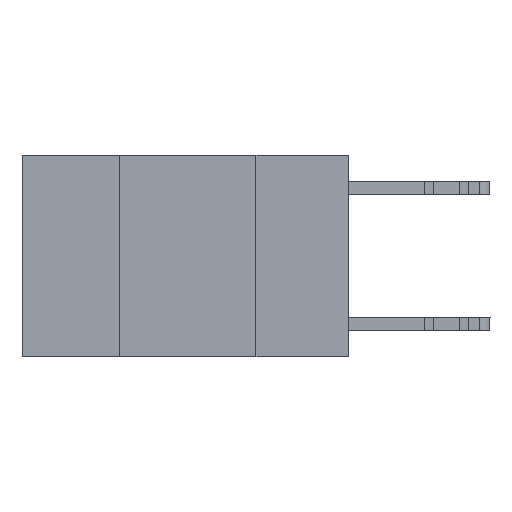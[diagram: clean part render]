
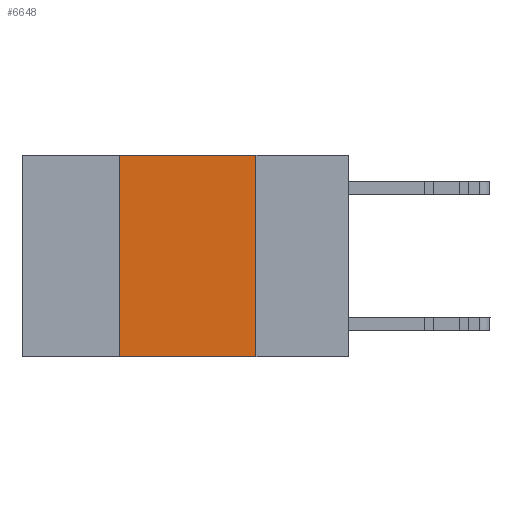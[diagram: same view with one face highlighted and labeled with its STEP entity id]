
A CAD part, left-side view. The second image highlights one B-rep face of the part: STEP entity #6648.
In plain terms, the highlighted planar face has unit normal (-1, 0, 0).
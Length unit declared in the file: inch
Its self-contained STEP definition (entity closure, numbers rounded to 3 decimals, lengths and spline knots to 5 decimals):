
#699 = LINE ( 'NONE', #27373, #13231 ) ;
#2178 = FACE_OUTER_BOUND ( 'NONE', #12333, .T. ) ;
#2464 = VERTEX_POINT ( 'NONE', #16812 ) ;
#3561 = DIRECTION ( 'NONE',  ( 0., 0., 1. ) ) ;
#5407 = VECTOR ( 'NONE', #8042, 39.37008 ) ;
#5435 = LINE ( 'NONE', #5542, #5407 ) ;
#5542 = CARTESIAN_POINT ( 'NONE',  ( 0., 0.17, 0. ) ) ;
#6648 = ADVANCED_FACE ( 'NONE', ( #2178 ), #23026, .F. ) ;
#8042 = DIRECTION ( 'NONE',  ( 0., 0., -1. ) ) ;
#11123 = VERTEX_POINT ( 'NONE', #26654 ) ;
#11436 = EDGE_CURVE ( 'NONE', #31077, #23239, #5435, .T. ) ;
#12333 = EDGE_LOOP ( 'NONE', ( #30022, #15157, #30770, #29256 ) ) ;
#13231 = VECTOR ( 'NONE', #15193, 39.37008 ) ;
#15157 = ORIENTED_EDGE ( 'NONE', *, *, #19989, .F. ) ;
#15193 = DIRECTION ( 'NONE',  ( 0., -1., 0. ) ) ;
#16106 = EDGE_CURVE ( 'NONE', #11123, #2464, #21958, .T. ) ;
#16633 = DIRECTION ( 'NONE',  ( 0., -1., 0. ) ) ;
#16812 = CARTESIAN_POINT ( 'NONE',  ( 0., 0.42, 0. ) ) ;
#17839 = CARTESIAN_POINT ( 'NONE',  ( 0., 0.17, 0. ) ) ;
#18481 = CARTESIAN_POINT ( 'NONE',  ( 0., 0.42, 0. ) ) ;
#19989 = EDGE_CURVE ( 'NONE', #2464, #31077, #699, .T. ) ;
#20414 = EDGE_CURVE ( 'NONE', #11123, #23239, #21357, .T. ) ;
#20572 = VECTOR ( 'NONE', #16633, 39.37008 ) ;
#21357 = LINE ( 'NONE', #23924, #20572 ) ;
#21958 = LINE ( 'NONE', #18481, #28351 ) ;
#22616 = DIRECTION ( 'NONE',  ( 0., 0., -1. ) ) ;
#22677 = DIRECTION ( 'NONE',  ( 1., 0., 0. ) ) ;
#23026 = PLANE ( 'NONE',  #29255 ) ;
#23054 = CARTESIAN_POINT ( 'NONE',  ( 0., 0.6, 0. ) ) ;
#23239 = VERTEX_POINT ( 'NONE', #31623 ) ;
#23924 = CARTESIAN_POINT ( 'NONE',  ( 0., 0.6, -0.37 ) ) ;
#26654 = CARTESIAN_POINT ( 'NONE',  ( 0., 0.42, -0.37 ) ) ;
#27373 = CARTESIAN_POINT ( 'NONE',  ( 0., 0.6, 0. ) ) ;
#28351 = VECTOR ( 'NONE', #3561, 39.37008 ) ;
#29255 = AXIS2_PLACEMENT_3D ( 'NONE', #23054, #22677, #22616 ) ;
#29256 = ORIENTED_EDGE ( 'NONE', *, *, #20414, .T. ) ;
#30022 = ORIENTED_EDGE ( 'NONE', *, *, #11436, .F. ) ;
#30770 = ORIENTED_EDGE ( 'NONE', *, *, #16106, .F. ) ;
#31077 = VERTEX_POINT ( 'NONE', #17839 ) ;
#31623 = CARTESIAN_POINT ( 'NONE',  ( 0., 0.17, -0.37 ) ) ;
